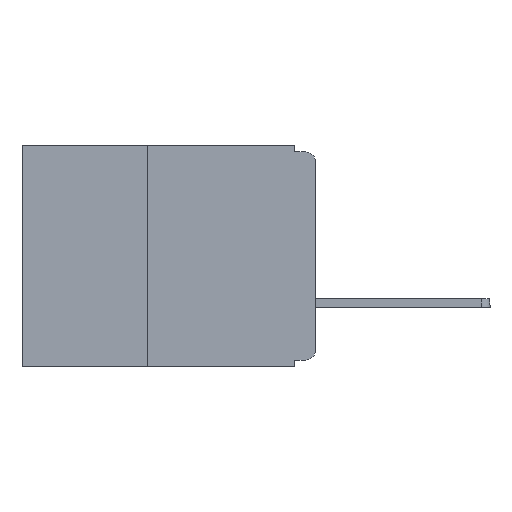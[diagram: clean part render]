
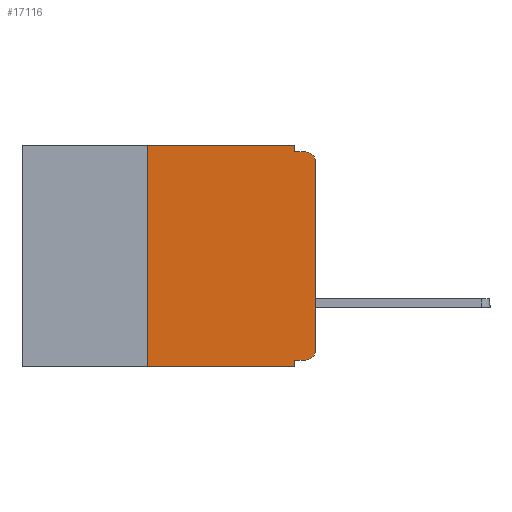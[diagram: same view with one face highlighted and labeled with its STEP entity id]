
A CAD part, left-side view. The second image highlights one B-rep face of the part: STEP entity #17116.
In plain terms, the highlighted planar face has unit normal (-1, 0, 0).
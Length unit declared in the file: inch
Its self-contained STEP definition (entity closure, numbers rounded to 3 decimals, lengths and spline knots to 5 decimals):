
#207 = VERTEX_POINT ( 'NONE', #28421 ) ;
#1139 = EDGE_CURVE ( 'NONE', #14360, #5484, #31941, .T. ) ;
#1283 = CARTESIAN_POINT ( 'NONE',  ( 0., 0.031, -0.01 ) ) ;
#3112 = ORIENTED_EDGE ( 'NONE', *, *, #6813, .T. ) ;
#3530 = VECTOR ( 'NONE', #32299, 39.37008 ) ;
#3668 = LINE ( 'NONE', #28789, #24651 ) ;
#4078 = CARTESIAN_POINT ( 'NONE',  ( 0., 0.437, 0. ) ) ;
#4153 = CIRCLE ( 'NONE', #20774, 0.015 ) ;
#4787 = VERTEX_POINT ( 'NONE', #12636 ) ;
#4966 = FACE_OUTER_BOUND ( 'NONE', #5505, .T. ) ;
#5377 = LINE ( 'NONE', #8183, #31387 ) ;
#5458 = CARTESIAN_POINT ( 'NONE',  ( 0., 0.015, -0.305 ) ) ;
#5484 = VERTEX_POINT ( 'NONE', #22356 ) ;
#5505 = EDGE_LOOP ( 'NONE', ( #3112, #28087, #15573, #27997, #5608, #27369, #27325, #26970, #12574, #12991 ) ) ;
#5608 = ORIENTED_EDGE ( 'NONE', *, *, #16862, .F. ) ;
#6198 = DIRECTION ( 'NONE',  ( 0., 0., 1. ) ) ;
#6813 = EDGE_CURVE ( 'NONE', #207, #30319, #25394, .T. ) ;
#7172 = CARTESIAN_POINT ( 'NONE',  ( 0., 0., -0.01 ) ) ;
#7953 = DIRECTION ( 'NONE',  ( 0., 0., -1. ) ) ;
#8183 = CARTESIAN_POINT ( 'NONE',  ( 0., 0.437, 0. ) ) ;
#10158 = LINE ( 'NONE', #21853, #16038 ) ;
#10346 = VERTEX_POINT ( 'NONE', #16723 ) ;
#10701 = DIRECTION ( 'NONE',  ( 0., -1., 0. ) ) ;
#11217 = VERTEX_POINT ( 'NONE', #30399 ) ;
#11559 = PLANE ( 'NONE',  #17089 ) ;
#11611 = AXIS2_PLACEMENT_3D ( 'NONE', #5458, #23130, #7953 ) ;
#11674 = DIRECTION ( 'NONE',  ( 1., 0., 0. ) ) ;
#11806 = VECTOR ( 'NONE', #24010, 39.37008 ) ;
#11901 = VECTOR ( 'NONE', #14234, 39.37008 ) ;
#12148 = DIRECTION ( 'NONE',  ( -1., 0., 0. ) ) ;
#12574 = ORIENTED_EDGE ( 'NONE', *, *, #1139, .F. ) ;
#12636 = CARTESIAN_POINT ( 'NONE',  ( 0., 0.015, -0.01 ) ) ;
#12991 = ORIENTED_EDGE ( 'NONE', *, *, #18677, .T. ) ;
#14234 = DIRECTION ( 'NONE',  ( 0., 0., 1. ) ) ;
#14360 = VERTEX_POINT ( 'NONE', #23783 ) ;
#14597 = VERTEX_POINT ( 'NONE', #19548 ) ;
#15573 = ORIENTED_EDGE ( 'NONE', *, *, #32305, .F. ) ;
#16038 = VECTOR ( 'NONE', #24392, 39.37008 ) ;
#16723 = CARTESIAN_POINT ( 'NONE',  ( 0., 0.25, -0.33 ) ) ;
#16862 = EDGE_CURVE ( 'NONE', #11217, #29300, #5377, .T. ) ;
#17050 = VERTEX_POINT ( 'NONE', #1283 ) ;
#17089 = AXIS2_PLACEMENT_3D ( 'NONE', #4078, #11674, #29382 ) ;
#17116 = ADVANCED_FACE ( 'NONE', ( #4966 ), #11559, .F. ) ;
#18497 = EDGE_CURVE ( 'NONE', #30319, #4787, #4153, .T. ) ;
#18677 = EDGE_CURVE ( 'NONE', #14360, #207, #29834, .T. ) ;
#19548 = CARTESIAN_POINT ( 'NONE',  ( 0., 0.031, -0.33 ) ) ;
#20527 = EDGE_CURVE ( 'NONE', #10346, #11217, #26558, .T. ) ;
#20774 = AXIS2_PLACEMENT_3D ( 'NONE', #27315, #12148, #29837 ) ;
#21237 = CARTESIAN_POINT ( 'NONE',  ( 0., 0., -0.025 ) ) ;
#21347 = CARTESIAN_POINT ( 'NONE',  ( 0., 0.25, -0.33 ) ) ;
#21853 = CARTESIAN_POINT ( 'NONE',  ( 0., 0.031, 0. ) ) ;
#22003 = CARTESIAN_POINT ( 'NONE',  ( 0., 0., -0.32 ) ) ;
#22356 = CARTESIAN_POINT ( 'NONE',  ( 0., 0.031, -0.32 ) ) ;
#22599 = EDGE_CURVE ( 'NONE', #5484, #14597, #29556, .T. ) ;
#23130 = DIRECTION ( 'NONE',  ( -1., 0., 0. ) ) ;
#23783 = CARTESIAN_POINT ( 'NONE',  ( 0., 0.015, -0.32 ) ) ;
#24010 = DIRECTION ( 'NONE',  ( 0., 1., 0. ) ) ;
#24227 = EDGE_CURVE ( 'NONE', #10346, #14597, #3668, .T. ) ;
#24392 = DIRECTION ( 'NONE',  ( 0., 0., -1. ) ) ;
#24438 = VECTOR ( 'NONE', #29921, 39.37008 ) ;
#24651 = VECTOR ( 'NONE', #31283, 39.37008 ) ;
#25394 = LINE ( 'NONE', #29389, #11901 ) ;
#25783 = VECTOR ( 'NONE', #6198, 39.37008 ) ;
#26558 = LINE ( 'NONE', #21347, #25783 ) ;
#26970 = ORIENTED_EDGE ( 'NONE', *, *, #22599, .F. ) ;
#27315 = CARTESIAN_POINT ( 'NONE',  ( 0., 0.015, -0.025 ) ) ;
#27325 = ORIENTED_EDGE ( 'NONE', *, *, #24227, .T. ) ;
#27369 = ORIENTED_EDGE ( 'NONE', *, *, #20527, .F. ) ;
#27504 = CARTESIAN_POINT ( 'NONE',  ( 0., 0.031, -0.33 ) ) ;
#27997 = ORIENTED_EDGE ( 'NONE', *, *, #28387, .F. ) ;
#28087 = ORIENTED_EDGE ( 'NONE', *, *, #18497, .T. ) ;
#28387 = EDGE_CURVE ( 'NONE', #29300, #17050, #10158, .T. ) ;
#28421 = CARTESIAN_POINT ( 'NONE',  ( 0., 0., -0.305 ) ) ;
#28789 = CARTESIAN_POINT ( 'NONE',  ( 0., 0.437, -0.33 ) ) ;
#29300 = VERTEX_POINT ( 'NONE', #32270 ) ;
#29382 = DIRECTION ( 'NONE',  ( 0., 0., -1. ) ) ;
#29389 = CARTESIAN_POINT ( 'NONE',  ( 0., 0., 0. ) ) ;
#29556 = LINE ( 'NONE', #27504, #24438 ) ;
#29834 = CIRCLE ( 'NONE', #11611, 0.015 ) ;
#29837 = DIRECTION ( 'NONE',  ( 0., 0., -1. ) ) ;
#29921 = DIRECTION ( 'NONE',  ( 0., 0., -1. ) ) ;
#30319 = VERTEX_POINT ( 'NONE', #21237 ) ;
#30399 = CARTESIAN_POINT ( 'NONE',  ( 0., 0.25, 0. ) ) ;
#30405 = LINE ( 'NONE', #7172, #3530 ) ;
#31283 = DIRECTION ( 'NONE',  ( 0., -1., 0. ) ) ;
#31387 = VECTOR ( 'NONE', #10701, 39.37008 ) ;
#31941 = LINE ( 'NONE', #22003, #11806 ) ;
#32270 = CARTESIAN_POINT ( 'NONE',  ( 0., 0.031, 0. ) ) ;
#32299 = DIRECTION ( 'NONE',  ( 0., -1., 0. ) ) ;
#32305 = EDGE_CURVE ( 'NONE', #17050, #4787, #30405, .T. ) ;
